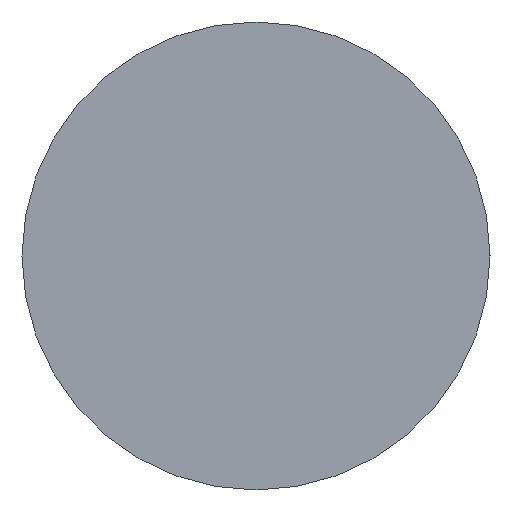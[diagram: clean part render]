
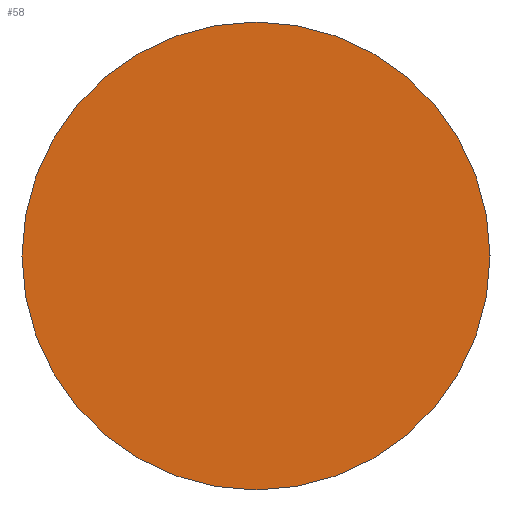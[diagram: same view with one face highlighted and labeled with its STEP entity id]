
A CAD part, left-side view. The second image highlights one B-rep face of the part: STEP entity #58.
In plain terms, the highlighted planar face has unit normal (-1, 0, 0).
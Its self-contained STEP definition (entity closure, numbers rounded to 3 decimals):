
#6 = AXIS2_PLACEMENT_3D ( 'NONE', #152, #140, #142 ) ;
#7 = VERTEX_POINT ( 'NONE', #158 ) ;
#9 = DIRECTION ( 'NONE',  ( 0., 0., -1. ) ) ;
#37 = ORIENTED_EDGE ( 'NONE', *, *, #82, .F. ) ;
#58 = ADVANCED_FACE ( 'NONE', ( #123 ), #133, .F. ) ;
#70 = DIRECTION ( 'NONE',  ( 0., 0., -1. ) ) ;
#78 = ORIENTED_EDGE ( 'NONE', *, *, #92, .F. ) ;
#79 = CIRCLE ( 'NONE', #103, 3.75 ) ;
#82 = EDGE_CURVE ( 'NONE', #161, #7, #79, .T. ) ;
#89 = CARTESIAN_POINT ( 'NONE',  ( 5.938, 0., 0. ) ) ;
#92 = EDGE_CURVE ( 'NONE', #7, #161, #157, .T. ) ;
#97 = EDGE_LOOP ( 'NONE', ( #78, #37 ) ) ;
#103 = AXIS2_PLACEMENT_3D ( 'NONE', #164, #162, #70 ) ;
#114 = CARTESIAN_POINT ( 'NONE',  ( 5.938, 0., -3.75 ) ) ;
#123 = FACE_OUTER_BOUND ( 'NONE', #97, .T. ) ;
#129 = AXIS2_PLACEMENT_3D ( 'NONE', #89, #160, #9 ) ;
#133 = PLANE ( 'NONE',  #129 ) ;
#140 = DIRECTION ( 'NONE',  ( 1., 0., 0. ) ) ;
#142 = DIRECTION ( 'NONE',  ( 0., 0., -1. ) ) ;
#152 = CARTESIAN_POINT ( 'NONE',  ( 5.938, 0., 0. ) ) ;
#157 = CIRCLE ( 'NONE', #6, 3.75 ) ;
#158 = CARTESIAN_POINT ( 'NONE',  ( 5.938, 0., 3.75 ) ) ;
#160 = DIRECTION ( 'NONE',  ( 1., 0., 0. ) ) ;
#161 = VERTEX_POINT ( 'NONE', #114 ) ;
#162 = DIRECTION ( 'NONE',  ( 1., 0., 0. ) ) ;
#164 = CARTESIAN_POINT ( 'NONE',  ( 5.938, 0., 0. ) ) ;
